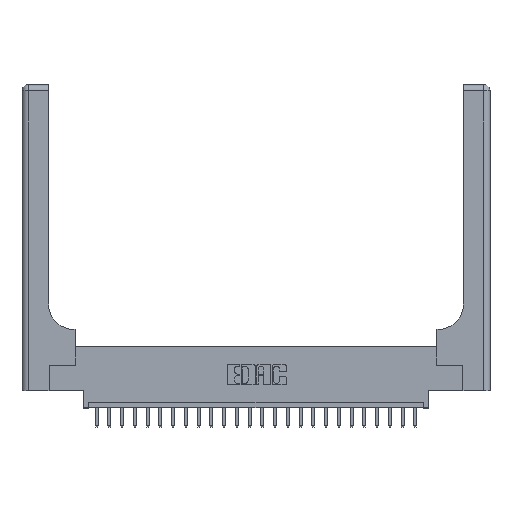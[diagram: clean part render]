
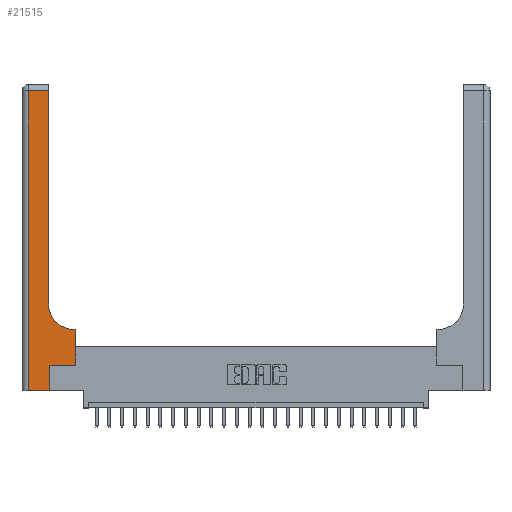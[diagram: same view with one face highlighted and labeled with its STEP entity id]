
A CAD part, top view. The second image highlights one B-rep face of the part: STEP entity #21515.
In plain terms, the highlighted planar face has unit normal (0, 0, 1).
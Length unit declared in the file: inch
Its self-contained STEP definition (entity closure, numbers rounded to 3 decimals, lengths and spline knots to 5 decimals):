
#797 = LINE ( 'NONE', #19828, #9053 ) ;
#1148 = CARTESIAN_POINT ( 'NONE',  ( 0., 0., 0.37 ) ) ;
#1666 = LINE ( 'NONE', #15558, #3064 ) ;
#2002 = VECTOR ( 'NONE', #8862, 39.37008 ) ;
#2071 = EDGE_CURVE ( 'NONE', #2192, #8377, #6217, .T. ) ;
#2107 = VERTEX_POINT ( 'NONE', #21200 ) ;
#2192 = VERTEX_POINT ( 'NONE', #10425 ) ;
#2532 = EDGE_CURVE ( 'NONE', #16429, #2192, #17762, .T. ) ;
#3064 = VECTOR ( 'NONE', #17123, 39.37008 ) ;
#3282 = CARTESIAN_POINT ( 'NONE',  ( 0.06, 2.94, 0.37 ) ) ;
#3340 = EDGE_LOOP ( 'NONE', ( #9106, #13831, #7915, #13726, #14399, #23751, #21074, #21627, #11225 ) ) ;
#3992 = CIRCLE ( 'NONE', #6908, 0.25 ) ;
#4350 = EDGE_CURVE ( 'NONE', #8377, #10788, #13016, .T. ) ;
#4764 = EDGE_CURVE ( 'NONE', #15121, #2107, #18224, .T. ) ;
#4998 = DIRECTION ( 'NONE',  ( 1., 0., 0. ) ) ;
#5078 = DIRECTION ( 'NONE',  ( 0., 0., -1. ) ) ;
#5230 = EDGE_CURVE ( 'NONE', #10788, #15121, #23300, .T. ) ;
#5424 = CARTESIAN_POINT ( 'NONE',  ( 0.06, 3., 0.37 ) ) ;
#5625 = VECTOR ( 'NONE', #21550, 39.37008 ) ;
#6217 = LINE ( 'NONE', #10127, #9668 ) ;
#6908 = AXIS2_PLACEMENT_3D ( 'NONE', #16051, #5078, #4998 ) ;
#7633 = CARTESIAN_POINT ( 'NONE',  ( 0.26, 0.6, 0.37 ) ) ;
#7915 = ORIENTED_EDGE ( 'NONE', *, *, #10455, .T. ) ;
#8101 = VECTOR ( 'NONE', #19954, 39.37008 ) ;
#8377 = VERTEX_POINT ( 'NONE', #15391 ) ;
#8862 = DIRECTION ( 'NONE',  ( 0., -1., 0. ) ) ;
#9053 = VECTOR ( 'NONE', #14761, 39.37008 ) ;
#9106 = ORIENTED_EDGE ( 'NONE', *, *, #13137, .T. ) ;
#9176 = DIRECTION ( 'NONE',  ( -1., 0., 0. ) ) ;
#9340 = CARTESIAN_POINT ( 'NONE',  ( 0.528, 0.25, 0.37 ) ) ;
#9668 = VECTOR ( 'NONE', #13900, 39.37008 ) ;
#9974 = PLANE ( 'NONE',  #12172 ) ;
#10127 = CARTESIAN_POINT ( 'NONE',  ( 0.265, 0., 0.37 ) ) ;
#10425 = CARTESIAN_POINT ( 'NONE',  ( 0.265, 0., 0.37 ) ) ;
#10455 = EDGE_CURVE ( 'NONE', #16832, #16429, #14036, .T. ) ;
#10788 = VERTEX_POINT ( 'NONE', #14254 ) ;
#11225 = ORIENTED_EDGE ( 'NONE', *, *, #21633, .T. ) ;
#11831 = CARTESIAN_POINT ( 'NONE',  ( 0., 3., 0.37 ) ) ;
#11836 = VECTOR ( 'NONE', #9176, 39.37008 ) ;
#12138 = VERTEX_POINT ( 'NONE', #22878 ) ;
#12172 = AXIS2_PLACEMENT_3D ( 'NONE', #11831, #21055, #22974 ) ;
#12398 = VERTEX_POINT ( 'NONE', #23665 ) ;
#13016 = LINE ( 'NONE', #20032, #8101 ) ;
#13137 = EDGE_CURVE ( 'NONE', #12138, #12398, #1666, .T. ) ;
#13383 = EDGE_CURVE ( 'NONE', #12398, #16832, #797, .T. ) ;
#13726 = ORIENTED_EDGE ( 'NONE', *, *, #2532, .T. ) ;
#13831 = ORIENTED_EDGE ( 'NONE', *, *, #13383, .T. ) ;
#13900 = DIRECTION ( 'NONE',  ( 0., 1., 0. ) ) ;
#14036 = LINE ( 'NONE', #5424, #2002 ) ;
#14254 = CARTESIAN_POINT ( 'NONE',  ( 0.528, 0.25, 0.37 ) ) ;
#14399 = ORIENTED_EDGE ( 'NONE', *, *, #2071, .T. ) ;
#14761 = DIRECTION ( 'NONE',  ( -1., 0., 0. ) ) ;
#14915 = DIRECTION ( 'NONE',  ( 0., 1., 0. ) ) ;
#15121 = VERTEX_POINT ( 'NONE', #15346 ) ;
#15346 = CARTESIAN_POINT ( 'NONE',  ( 0.528, 0.6, 0.37 ) ) ;
#15391 = CARTESIAN_POINT ( 'NONE',  ( 0.265, 0.25, 0.37 ) ) ;
#15496 = FACE_OUTER_BOUND ( 'NONE', #3340, .T. ) ;
#15558 = CARTESIAN_POINT ( 'NONE',  ( 0.26, 3., 0.37 ) ) ;
#16051 = CARTESIAN_POINT ( 'NONE',  ( 0.51, 0.85, 0.37 ) ) ;
#16429 = VERTEX_POINT ( 'NONE', #17977 ) ;
#16832 = VERTEX_POINT ( 'NONE', #3282 ) ;
#17123 = DIRECTION ( 'NONE',  ( 0., 1., 0. ) ) ;
#17762 = LINE ( 'NONE', #1148, #5625 ) ;
#17977 = CARTESIAN_POINT ( 'NONE',  ( 0.06, 0., 0.37 ) ) ;
#18224 = LINE ( 'NONE', #7633, #11836 ) ;
#18478 = VECTOR ( 'NONE', #14915, 39.37008 ) ;
#19828 = CARTESIAN_POINT ( 'NONE',  ( 0., 2.94, 0.37 ) ) ;
#19954 = DIRECTION ( 'NONE',  ( 1., 0., 0. ) ) ;
#20032 = CARTESIAN_POINT ( 'NONE',  ( 0.265, 0.25, 0.37 ) ) ;
#21055 = DIRECTION ( 'NONE',  ( 0., 0., -1. ) ) ;
#21074 = ORIENTED_EDGE ( 'NONE', *, *, #5230, .T. ) ;
#21200 = CARTESIAN_POINT ( 'NONE',  ( 0.51, 0.6, 0.37 ) ) ;
#21515 = ADVANCED_FACE ( 'NONE', ( #15496 ), #9974, .F. ) ;
#21550 = DIRECTION ( 'NONE',  ( 1., 0., 0. ) ) ;
#21627 = ORIENTED_EDGE ( 'NONE', *, *, #4764, .T. ) ;
#21633 = EDGE_CURVE ( 'NONE', #2107, #12138, #3992, .T. ) ;
#22878 = CARTESIAN_POINT ( 'NONE',  ( 0.26, 0.85, 0.37 ) ) ;
#22974 = DIRECTION ( 'NONE',  ( -1., 0., 0. ) ) ;
#23300 = LINE ( 'NONE', #9340, #18478 ) ;
#23665 = CARTESIAN_POINT ( 'NONE',  ( 0.26, 2.94, 0.37 ) ) ;
#23751 = ORIENTED_EDGE ( 'NONE', *, *, #4350, .T. ) ;
